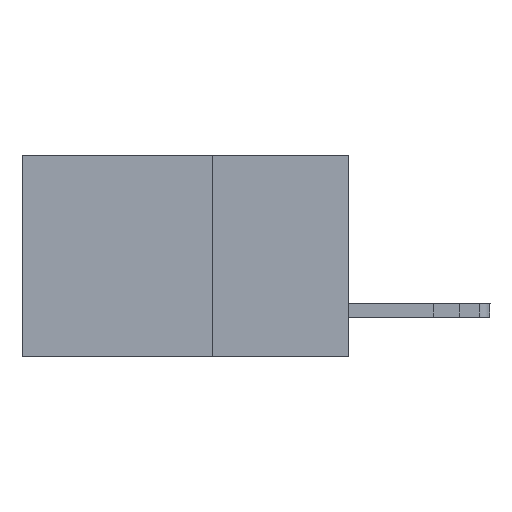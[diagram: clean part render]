
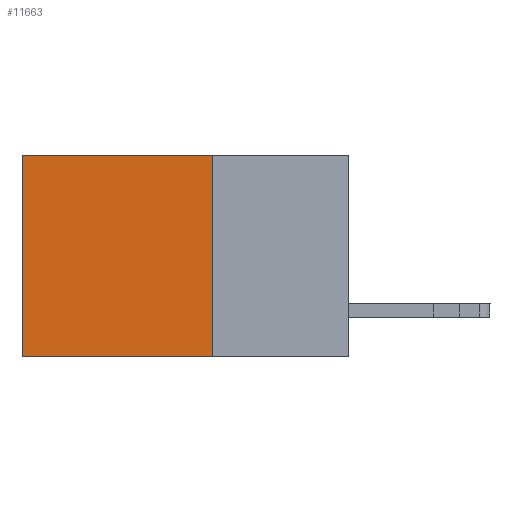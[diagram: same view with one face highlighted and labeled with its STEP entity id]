
A CAD part, left-side view. The second image highlights one B-rep face of the part: STEP entity #11663.
In plain terms, the highlighted planar face has unit normal (-1, 0, 0).
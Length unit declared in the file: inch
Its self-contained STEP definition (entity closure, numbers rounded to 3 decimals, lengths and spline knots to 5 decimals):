
#929 = CARTESIAN_POINT ( 'NONE',  ( 0.298, 0.6, 0. ) ) ;
#1009 = PLANE ( 'NONE',  #6184 ) ;
#1630 = ORIENTED_EDGE ( 'NONE', *, *, #14417, .F. ) ;
#1741 = EDGE_LOOP ( 'NONE', ( #5648, #6925, #1630, #4888 ) ) ;
#2563 = VERTEX_POINT ( 'NONE', #8611 ) ;
#2686 = VECTOR ( 'NONE', #12232, 39.37008 ) ;
#2800 = VERTEX_POINT ( 'NONE', #4757 ) ;
#2912 = EDGE_CURVE ( 'NONE', #2800, #2563, #3055, .T. ) ;
#3055 = LINE ( 'NONE', #929, #13145 ) ;
#3589 = DIRECTION ( 'NONE',  ( 0., 1., 0. ) ) ;
#3642 = CARTESIAN_POINT ( 'NONE',  ( 0.298, 0.25, -0.37 ) ) ;
#4092 = DIRECTION ( 'NONE',  ( 0., 0., -1. ) ) ;
#4270 = VERTEX_POINT ( 'NONE', #8391 ) ;
#4390 = CARTESIAN_POINT ( 'NONE',  ( 0.298, 0.25, 0. ) ) ;
#4625 = CARTESIAN_POINT ( 'NONE',  ( 0.298, 0.25, 0. ) ) ;
#4757 = CARTESIAN_POINT ( 'NONE',  ( 0.298, 0.6, 0. ) ) ;
#4798 = CARTESIAN_POINT ( 'NONE',  ( 0.298, 0.25, 0. ) ) ;
#4888 = ORIENTED_EDGE ( 'NONE', *, *, #11316, .T. ) ;
#5648 = ORIENTED_EDGE ( 'NONE', *, *, #2912, .T. ) ;
#6184 = AXIS2_PLACEMENT_3D ( 'NONE', #4390, #8864, #7300 ) ;
#6925 = ORIENTED_EDGE ( 'NONE', *, *, #13657, .F. ) ;
#7300 = DIRECTION ( 'NONE',  ( 0., 0., -1. ) ) ;
#8391 = CARTESIAN_POINT ( 'NONE',  ( 0.298, 0.25, -0.37 ) ) ;
#8611 = CARTESIAN_POINT ( 'NONE',  ( 0.298, 0.6, -0.37 ) ) ;
#8835 = LINE ( 'NONE', #13342, #2686 ) ;
#8864 = DIRECTION ( 'NONE',  ( 1., 0., 0. ) ) ;
#9176 = LINE ( 'NONE', #4625, #11141 ) ;
#10639 = DIRECTION ( 'NONE',  ( 0., 1., 0. ) ) ;
#11141 = VECTOR ( 'NONE', #3589, 39.37008 ) ;
#11316 = EDGE_CURVE ( 'NONE', #12767, #2800, #9176, .T. ) ;
#11663 = ADVANCED_FACE ( 'NONE', ( #13308 ), #1009, .F. ) ;
#11821 = LINE ( 'NONE', #3642, #12818 ) ;
#12232 = DIRECTION ( 'NONE',  ( 0., 0., -1. ) ) ;
#12767 = VERTEX_POINT ( 'NONE', #4798 ) ;
#12818 = VECTOR ( 'NONE', #10639, 39.37008 ) ;
#13145 = VECTOR ( 'NONE', #4092, 39.37008 ) ;
#13308 = FACE_OUTER_BOUND ( 'NONE', #1741, .T. ) ;
#13342 = CARTESIAN_POINT ( 'NONE',  ( 0.298, 0.25, 0. ) ) ;
#13657 = EDGE_CURVE ( 'NONE', #4270, #2563, #11821, .T. ) ;
#14417 = EDGE_CURVE ( 'NONE', #12767, #4270, #8835, .T. ) ;
